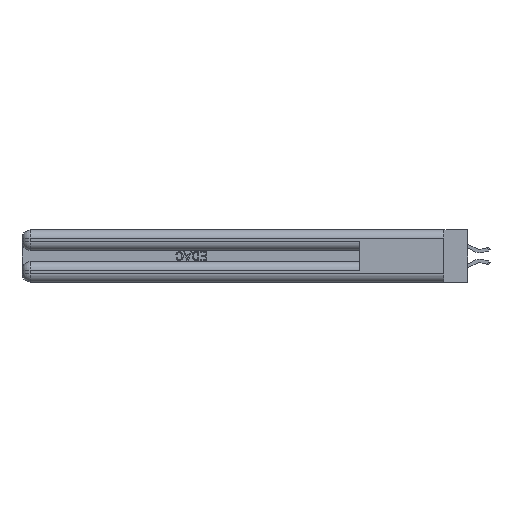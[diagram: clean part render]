
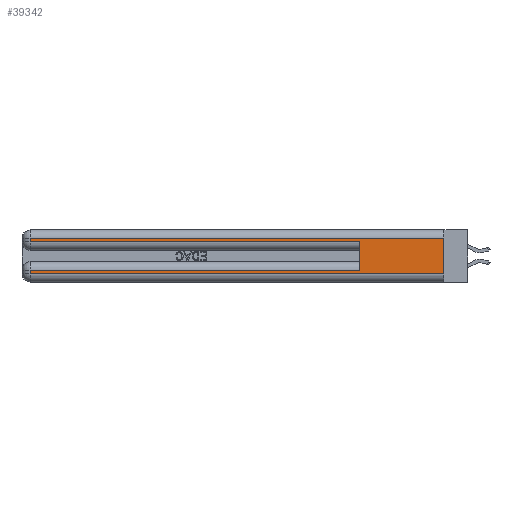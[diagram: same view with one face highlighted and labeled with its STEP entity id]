
A CAD part, left-side view. The second image highlights one B-rep face of the part: STEP entity #39342.
In plain terms, the highlighted planar face has unit normal (-1, 0, 0).
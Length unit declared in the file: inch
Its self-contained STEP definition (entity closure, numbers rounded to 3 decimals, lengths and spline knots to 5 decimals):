
#3935 = EDGE_CURVE ( 'NONE', #25110, #13768, #41919, .T. ) ;
#4466 = ORIENTED_EDGE ( 'NONE', *, *, #14181, .T. ) ;
#5594 = VECTOR ( 'NONE', #34864, 39.37008 ) ;
#5832 = DIRECTION ( 'NONE',  ( 0., -1., 0. ) ) ;
#6118 = ORIENTED_EDGE ( 'NONE', *, *, #3935, .F. ) ;
#6891 = VERTEX_POINT ( 'NONE', #19749 ) ;
#7107 = CARTESIAN_POINT ( 'NONE',  ( 0., 2.94, 0.085 ) ) ;
#7224 = ORIENTED_EDGE ( 'NONE', *, *, #31551, .T. ) ;
#8136 = CARTESIAN_POINT ( 'NONE',  ( 0., 0.6, 0.145 ) ) ;
#8380 = VERTEX_POINT ( 'NONE', #11622 ) ;
#8665 = PLANE ( 'NONE',  #21446 ) ;
#9185 = VECTOR ( 'NONE', #27437, 39.37008 ) ;
#9620 = CARTESIAN_POINT ( 'NONE',  ( 0., 2.94, 0.285 ) ) ;
#10459 = ORIENTED_EDGE ( 'NONE', *, *, #13911, .T. ) ;
#10546 = LINE ( 'NONE', #41159, #27664 ) ;
#11400 = LINE ( 'NONE', #36461, #37500 ) ;
#11622 = CARTESIAN_POINT ( 'NONE',  ( 0., 2.94, 0.06 ) ) ;
#12096 = ORIENTED_EDGE ( 'NONE', *, *, #17694, .F. ) ;
#12194 = CARTESIAN_POINT ( 'NONE',  ( 0., 0., 0.37 ) ) ;
#13359 = CARTESIAN_POINT ( 'NONE',  ( 0., 0.6, 0.085 ) ) ;
#13768 = VERTEX_POINT ( 'NONE', #29029 ) ;
#13911 = EDGE_CURVE ( 'NONE', #17286, #21257, #39383, .T. ) ;
#14181 = EDGE_CURVE ( 'NONE', #25110, #17259, #10546, .T. ) ;
#14611 = DIRECTION ( 'NONE',  ( 0., 0., -1. ) ) ;
#15341 = ORIENTED_EDGE ( 'NONE', *, *, #42305, .T. ) ;
#15727 = DIRECTION ( 'NONE',  ( 1., 0., 0. ) ) ;
#17259 = VERTEX_POINT ( 'NONE', #7107 ) ;
#17286 = VERTEX_POINT ( 'NONE', #37849 ) ;
#17694 = EDGE_CURVE ( 'NONE', #17286, #6891, #11400, .T. ) ;
#19749 = CARTESIAN_POINT ( 'NONE',  ( 0., 0., 0.06 ) ) ;
#21257 = VERTEX_POINT ( 'NONE', #41125 ) ;
#21446 = AXIS2_PLACEMENT_3D ( 'NONE', #12194, #15727, #39422 ) ;
#21629 = VECTOR ( 'NONE', #14611, 39.37008 ) ;
#24222 = EDGE_CURVE ( 'NONE', #8380, #6891, #38535, .T. ) ;
#25110 = VERTEX_POINT ( 'NONE', #13359 ) ;
#25437 = DIRECTION ( 'NONE',  ( 0., 0., 1. ) ) ;
#26386 = CARTESIAN_POINT ( 'NONE',  ( 0., 0., 0.31 ) ) ;
#27437 = DIRECTION ( 'NONE',  ( 0., -1., 0. ) ) ;
#27664 = VECTOR ( 'NONE', #27670, 39.37008 ) ;
#27670 = DIRECTION ( 'NONE',  ( 0., 1., 0. ) ) ;
#28092 = CARTESIAN_POINT ( 'NONE',  ( 0., 2.94, 0.37 ) ) ;
#28466 = LINE ( 'NONE', #44282, #9185 ) ;
#29029 = CARTESIAN_POINT ( 'NONE',  ( 0., 0.6, 0.285 ) ) ;
#29765 = DIRECTION ( 'NONE',  ( 0., 1., 0. ) ) ;
#29780 = CARTESIAN_POINT ( 'NONE',  ( 0., 0., 0.06 ) ) ;
#31551 = EDGE_CURVE ( 'NONE', #42674, #13768, #28466, .T. ) ;
#32927 = VECTOR ( 'NONE', #25437, 39.37008 ) ;
#34864 = DIRECTION ( 'NONE',  ( 0., 0., -1. ) ) ;
#35510 = ORIENTED_EDGE ( 'NONE', *, *, #39800, .T. ) ;
#36461 = CARTESIAN_POINT ( 'NONE',  ( 0., 0., 0.37 ) ) ;
#37500 = VECTOR ( 'NONE', #39891, 39.37008 ) ;
#37849 = CARTESIAN_POINT ( 'NONE',  ( 0., 0., 0.31 ) ) ;
#38304 = VECTOR ( 'NONE', #29765, 39.37008 ) ;
#38535 = LINE ( 'NONE', #29780, #43268 ) ;
#39292 = EDGE_LOOP ( 'NONE', ( #12096, #10459, #35510, #7224, #6118, #4466, #15341, #42355 ) ) ;
#39342 = ADVANCED_FACE ( 'NONE', ( #39640 ), #8665, .F. ) ;
#39383 = LINE ( 'NONE', #26386, #38304 ) ;
#39422 = DIRECTION ( 'NONE',  ( 0., 0., -1. ) ) ;
#39594 = LINE ( 'NONE', #28092, #21629 ) ;
#39640 = FACE_OUTER_BOUND ( 'NONE', #39292, .T. ) ;
#39800 = EDGE_CURVE ( 'NONE', #21257, #42674, #39594, .T. ) ;
#39891 = DIRECTION ( 'NONE',  ( 0., 0., -1. ) ) ;
#41125 = CARTESIAN_POINT ( 'NONE',  ( 0., 2.94, 0.31 ) ) ;
#41159 = CARTESIAN_POINT ( 'NONE',  ( 0., 0., 0.085 ) ) ;
#41568 = CARTESIAN_POINT ( 'NONE',  ( 0., 2.94, 0.37 ) ) ;
#41903 = LINE ( 'NONE', #41568, #5594 ) ;
#41919 = LINE ( 'NONE', #8136, #32927 ) ;
#42305 = EDGE_CURVE ( 'NONE', #17259, #8380, #41903, .T. ) ;
#42355 = ORIENTED_EDGE ( 'NONE', *, *, #24222, .T. ) ;
#42674 = VERTEX_POINT ( 'NONE', #9620 ) ;
#43268 = VECTOR ( 'NONE', #5832, 39.37008 ) ;
#44282 = CARTESIAN_POINT ( 'NONE',  ( 0., 0., 0.285 ) ) ;
